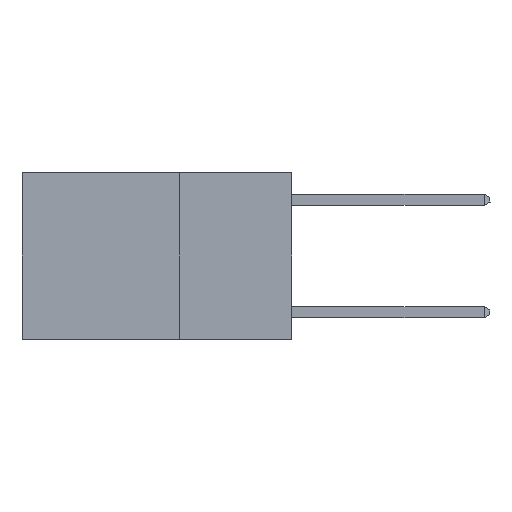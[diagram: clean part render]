
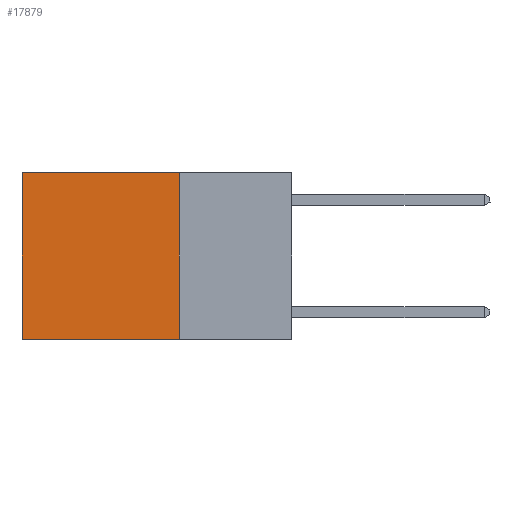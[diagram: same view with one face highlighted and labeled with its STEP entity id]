
A CAD part, left-side view. The second image highlights one B-rep face of the part: STEP entity #17879.
In plain terms, the highlighted planar face has unit normal (-1, 0, 0).
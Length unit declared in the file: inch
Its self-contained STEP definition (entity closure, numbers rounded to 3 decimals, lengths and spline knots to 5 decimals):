
#2572 = EDGE_LOOP ( 'NONE', ( #9537, #5134, #2881, #18966 ) ) ;
#2881 = ORIENTED_EDGE ( 'NONE', *, *, #7971, .F. ) ;
#2956 = PLANE ( 'NONE',  #7787 ) ;
#3455 = EDGE_CURVE ( 'NONE', #14199, #11728, #9338, .T. ) ;
#5134 = ORIENTED_EDGE ( 'NONE', *, *, #3455, .F. ) ;
#5365 = VECTOR ( 'NONE', #15980, 39.37008 ) ;
#5544 = DIRECTION ( 'NONE',  ( 0., 0., -1. ) ) ;
#5604 = CARTESIAN_POINT ( 'NONE',  ( 0.2625, 0.25, -0.37 ) ) ;
#7213 = VECTOR ( 'NONE', #10632, 39.37008 ) ;
#7480 = DIRECTION ( 'NONE',  ( 1., 0., 0. ) ) ;
#7571 = CARTESIAN_POINT ( 'NONE',  ( 0.2625, 0.25, -0.37 ) ) ;
#7787 = AXIS2_PLACEMENT_3D ( 'NONE', #16376, #7480, #17864 ) ;
#7971 = EDGE_CURVE ( 'NONE', #14150, #14199, #14897, .T. ) ;
#9134 = CARTESIAN_POINT ( 'NONE',  ( 0.2625, 0.25, 0. ) ) ;
#9338 = LINE ( 'NONE', #5604, #5365 ) ;
#9537 = ORIENTED_EDGE ( 'NONE', *, *, #18764, .T. ) ;
#10632 = DIRECTION ( 'NONE',  ( 0., 1., 0. ) ) ;
#10889 = FACE_OUTER_BOUND ( 'NONE', #2572, .T. ) ;
#11291 = EDGE_CURVE ( 'NONE', #14150, #13421, #14640, .T. ) ;
#11728 = VERTEX_POINT ( 'NONE', #16170 ) ;
#11746 = CARTESIAN_POINT ( 'NONE',  ( 0.2625, 0.6, 0. ) ) ;
#11755 = LINE ( 'NONE', #17062, #14765 ) ;
#13352 = CARTESIAN_POINT ( 'NONE',  ( 0.2625, 0.25, 0. ) ) ;
#13421 = VERTEX_POINT ( 'NONE', #11746 ) ;
#14117 = DIRECTION ( 'NONE',  ( 0., 0., -1. ) ) ;
#14150 = VERTEX_POINT ( 'NONE', #13352 ) ;
#14199 = VERTEX_POINT ( 'NONE', #7571 ) ;
#14429 = VECTOR ( 'NONE', #5544, 39.37008 ) ;
#14640 = LINE ( 'NONE', #9134, #7213 ) ;
#14765 = VECTOR ( 'NONE', #14117, 39.37008 ) ;
#14897 = LINE ( 'NONE', #17357, #14429 ) ;
#15980 = DIRECTION ( 'NONE',  ( 0., 1., 0. ) ) ;
#16170 = CARTESIAN_POINT ( 'NONE',  ( 0.2625, 0.6, -0.37 ) ) ;
#16376 = CARTESIAN_POINT ( 'NONE',  ( 0.2625, 0.25, 0. ) ) ;
#17062 = CARTESIAN_POINT ( 'NONE',  ( 0.2625, 0.6, 0. ) ) ;
#17357 = CARTESIAN_POINT ( 'NONE',  ( 0.2625, 0.25, 0. ) ) ;
#17864 = DIRECTION ( 'NONE',  ( 0., 0., -1. ) ) ;
#17879 = ADVANCED_FACE ( 'NONE', ( #10889 ), #2956, .F. ) ;
#18764 = EDGE_CURVE ( 'NONE', #13421, #11728, #11755, .T. ) ;
#18966 = ORIENTED_EDGE ( 'NONE', *, *, #11291, .T. ) ;
